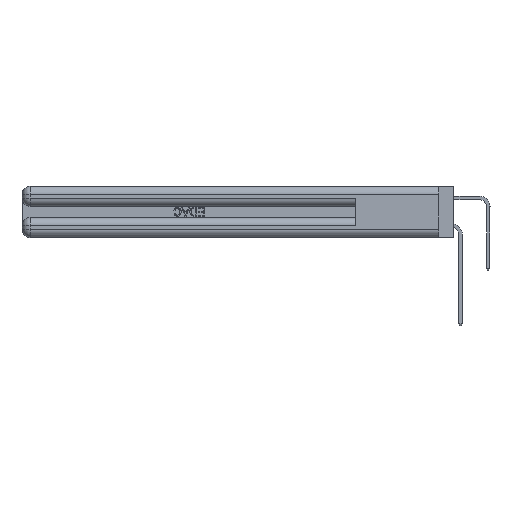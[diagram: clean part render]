
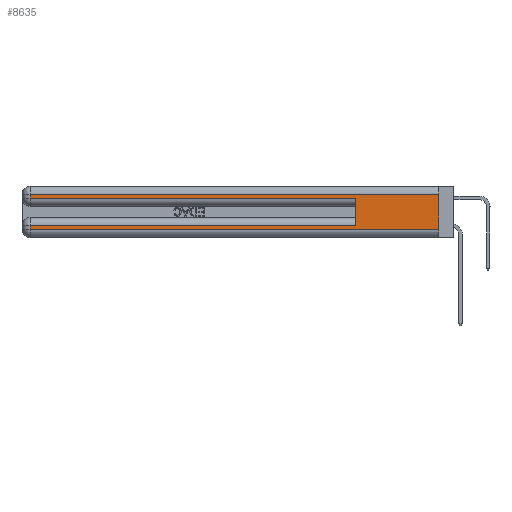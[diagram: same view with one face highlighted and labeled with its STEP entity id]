
A CAD part, left-side view. The second image highlights one B-rep face of the part: STEP entity #8635.
In plain terms, the highlighted planar face has unit normal (-1, 0, 0).
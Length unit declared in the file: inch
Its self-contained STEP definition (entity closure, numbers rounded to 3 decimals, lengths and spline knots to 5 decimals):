
#224 = EDGE_CURVE ( 'NONE', #14970, #35531, #26767, .T. ) ;
#1883 = ORIENTED_EDGE ( 'NONE', *, *, #29942, .T. ) ;
#2933 = VERTEX_POINT ( 'NONE', #13510 ) ;
#3535 = ORIENTED_EDGE ( 'NONE', *, *, #224, .T. ) ;
#4683 = CARTESIAN_POINT ( 'NONE',  ( 0., 0.6, 0.085 ) ) ;
#6329 = VECTOR ( 'NONE', #18217, 39.37008 ) ;
#6522 = ORIENTED_EDGE ( 'NONE', *, *, #9603, .T. ) ;
#7242 = LINE ( 'NONE', #18046, #44438 ) ;
#7404 = EDGE_CURVE ( 'NONE', #2933, #48910, #39857, .T. ) ;
#7577 = VECTOR ( 'NONE', #15980, 39.37008 ) ;
#8635 = ADVANCED_FACE ( 'NONE', ( #26578 ), #16173, .F. ) ;
#9120 = CARTESIAN_POINT ( 'NONE',  ( 0., 2.94, 0.31 ) ) ;
#9163 = DIRECTION ( 'NONE',  ( 0., 0., 1. ) ) ;
#9603 = EDGE_CURVE ( 'NONE', #22810, #23561, #7242, .T. ) ;
#10229 = CARTESIAN_POINT ( 'NONE',  ( 0., 0., 0.285 ) ) ;
#10394 = CARTESIAN_POINT ( 'NONE',  ( 0., 0., 0.06 ) ) ;
#10474 = VECTOR ( 'NONE', #44190, 39.37008 ) ;
#12830 = EDGE_CURVE ( 'NONE', #48910, #24175, #37017, .T. ) ;
#13023 = VECTOR ( 'NONE', #30272, 39.37008 ) ;
#13510 = CARTESIAN_POINT ( 'NONE',  ( 0., 0., 0.31 ) ) ;
#13522 = CARTESIAN_POINT ( 'NONE',  ( 0., 0., 0.31 ) ) ;
#14802 = VERTEX_POINT ( 'NONE', #39231 ) ;
#14970 = VERTEX_POINT ( 'NONE', #28663 ) ;
#15980 = DIRECTION ( 'NONE',  ( 0., 0., -1. ) ) ;
#16173 = PLANE ( 'NONE',  #32951 ) ;
#16375 = ORIENTED_EDGE ( 'NONE', *, *, #7404, .T. ) ;
#18046 = CARTESIAN_POINT ( 'NONE',  ( 0., 0., 0.085 ) ) ;
#18217 = DIRECTION ( 'NONE',  ( 0., -1., 0. ) ) ;
#19398 = EDGE_CURVE ( 'NONE', #2933, #35531, #23306, .T. ) ;
#21597 = EDGE_CURVE ( 'NONE', #22810, #14802, #38535, .T. ) ;
#22810 = VERTEX_POINT ( 'NONE', #4683 ) ;
#23306 = LINE ( 'NONE', #45480, #13023 ) ;
#23561 = VERTEX_POINT ( 'NONE', #40175 ) ;
#23875 = DIRECTION ( 'NONE',  ( 0., 0., -1. ) ) ;
#24175 = VERTEX_POINT ( 'NONE', #46770 ) ;
#26578 = FACE_OUTER_BOUND ( 'NONE', #28497, .T. ) ;
#26767 = LINE ( 'NONE', #10394, #6329 ) ;
#28113 = DIRECTION ( 'NONE',  ( 0., 0., -1. ) ) ;
#28281 = CARTESIAN_POINT ( 'NONE',  ( 0., 0.6, 0.145 ) ) ;
#28497 = EDGE_LOOP ( 'NONE', ( #45691, #16375, #40297, #1883, #34920, #6522, #47227, #3535 ) ) ;
#28663 = CARTESIAN_POINT ( 'NONE',  ( 0., 2.94, 0.06 ) ) ;
#29942 = EDGE_CURVE ( 'NONE', #24175, #14802, #45800, .T. ) ;
#30272 = DIRECTION ( 'NONE',  ( 0., 0., -1. ) ) ;
#32951 = AXIS2_PLACEMENT_3D ( 'NONE', #42895, #46772, #23875 ) ;
#34920 = ORIENTED_EDGE ( 'NONE', *, *, #21597, .F. ) ;
#35531 = VERTEX_POINT ( 'NONE', #38317 ) ;
#35890 = VECTOR ( 'NONE', #28113, 39.37008 ) ;
#36832 = VECTOR ( 'NONE', #40896, 39.37008 ) ;
#37017 = LINE ( 'NONE', #42722, #7577 ) ;
#37114 = LINE ( 'NONE', #47213, #35890 ) ;
#38317 = CARTESIAN_POINT ( 'NONE',  ( 0., 0., 0.06 ) ) ;
#38535 = LINE ( 'NONE', #28281, #46317 ) ;
#39231 = CARTESIAN_POINT ( 'NONE',  ( 0., 0.6, 0.285 ) ) ;
#39857 = LINE ( 'NONE', #13522, #10474 ) ;
#40175 = CARTESIAN_POINT ( 'NONE',  ( 0., 2.94, 0.085 ) ) ;
#40297 = ORIENTED_EDGE ( 'NONE', *, *, #12830, .T. ) ;
#40896 = DIRECTION ( 'NONE',  ( 0., -1., 0. ) ) ;
#41407 = EDGE_CURVE ( 'NONE', #23561, #14970, #37114, .T. ) ;
#42722 = CARTESIAN_POINT ( 'NONE',  ( 0., 2.94, 0.37 ) ) ;
#42895 = CARTESIAN_POINT ( 'NONE',  ( 0., 0., 0.37 ) ) ;
#44190 = DIRECTION ( 'NONE',  ( 0., 1., 0. ) ) ;
#44438 = VECTOR ( 'NONE', #48627, 39.37008 ) ;
#45480 = CARTESIAN_POINT ( 'NONE',  ( 0., 0., 0.37 ) ) ;
#45691 = ORIENTED_EDGE ( 'NONE', *, *, #19398, .F. ) ;
#45800 = LINE ( 'NONE', #10229, #36832 ) ;
#46317 = VECTOR ( 'NONE', #9163, 39.37008 ) ;
#46770 = CARTESIAN_POINT ( 'NONE',  ( 0., 2.94, 0.285 ) ) ;
#46772 = DIRECTION ( 'NONE',  ( 1., 0., 0. ) ) ;
#47213 = CARTESIAN_POINT ( 'NONE',  ( 0., 2.94, 0.37 ) ) ;
#47227 = ORIENTED_EDGE ( 'NONE', *, *, #41407, .T. ) ;
#48627 = DIRECTION ( 'NONE',  ( 0., 1., 0. ) ) ;
#48910 = VERTEX_POINT ( 'NONE', #9120 ) ;
